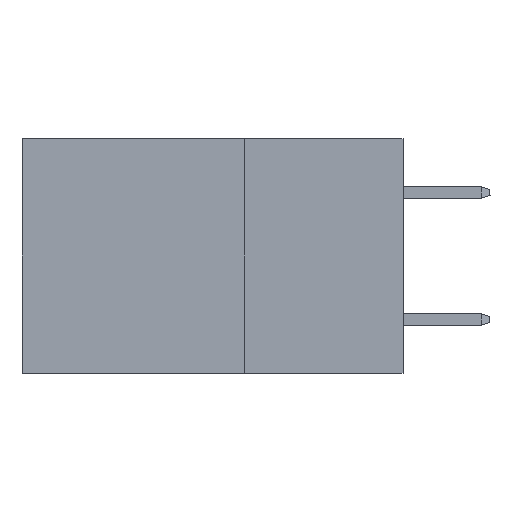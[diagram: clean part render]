
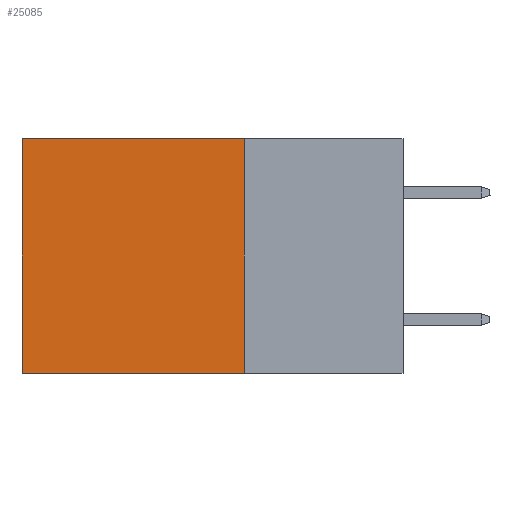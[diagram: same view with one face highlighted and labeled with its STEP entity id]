
A CAD part, left-side view. The second image highlights one B-rep face of the part: STEP entity #25085.
In plain terms, the highlighted planar face has unit normal (-1, 0, 0).
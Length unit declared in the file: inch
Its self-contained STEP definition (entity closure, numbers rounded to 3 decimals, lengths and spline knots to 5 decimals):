
#2461 = CARTESIAN_POINT ( 'NONE',  ( 0.2875, 0.6, -0.37 ) ) ;
#2779 = ORIENTED_EDGE ( 'NONE', *, *, #23482, .F. ) ;
#4397 = VERTEX_POINT ( 'NONE', #34480 ) ;
#4522 = DIRECTION ( 'NONE',  ( 0., 1., 0. ) ) ;
#4801 = CARTESIAN_POINT ( 'NONE',  ( 0.2875, 0.25, 0. ) ) ;
#5065 = LINE ( 'NONE', #26636, #22293 ) ;
#5544 = FACE_OUTER_BOUND ( 'NONE', #16501, .T. ) ;
#5665 = LINE ( 'NONE', #24556, #15319 ) ;
#6020 = CARTESIAN_POINT ( 'NONE',  ( 0.2875, 0.25, 0. ) ) ;
#7128 = VERTEX_POINT ( 'NONE', #9201 ) ;
#7500 = LINE ( 'NONE', #4801, #32509 ) ;
#9201 = CARTESIAN_POINT ( 'NONE',  ( 0.2875, 0.25, -0.37 ) ) ;
#9951 = ORIENTED_EDGE ( 'NONE', *, *, #18969, .F. ) ;
#11733 = ORIENTED_EDGE ( 'NONE', *, *, #13972, .T. ) ;
#11778 = VECTOR ( 'NONE', #14407, 39.37008 ) ;
#12647 = DIRECTION ( 'NONE',  ( 0., 0., -1. ) ) ;
#13736 = DIRECTION ( 'NONE',  ( 0., 0., -1. ) ) ;
#13972 = EDGE_CURVE ( 'NONE', #15903, #4397, #14052, .T. ) ;
#14052 = LINE ( 'NONE', #6020, #11778 ) ;
#14407 = DIRECTION ( 'NONE',  ( 0., 1., 0. ) ) ;
#15319 = VECTOR ( 'NONE', #16582, 39.37008 ) ;
#15903 = VERTEX_POINT ( 'NONE', #30292 ) ;
#16269 = PLANE ( 'NONE',  #17041 ) ;
#16460 = DIRECTION ( 'NONE',  ( 1., 0., 0. ) ) ;
#16501 = EDGE_LOOP ( 'NONE', ( #31914, #2779, #9951, #11733 ) ) ;
#16582 = DIRECTION ( 'NONE',  ( 0., 0., -1. ) ) ;
#17041 = AXIS2_PLACEMENT_3D ( 'NONE', #27297, #16460, #13736 ) ;
#18969 = EDGE_CURVE ( 'NONE', #15903, #7128, #7500, .T. ) ;
#22293 = VECTOR ( 'NONE', #4522, 39.37008 ) ;
#23482 = EDGE_CURVE ( 'NONE', #7128, #24217, #5065, .T. ) ;
#24217 = VERTEX_POINT ( 'NONE', #2461 ) ;
#24556 = CARTESIAN_POINT ( 'NONE',  ( 0.2875, 0.6, 0. ) ) ;
#25085 = ADVANCED_FACE ( 'NONE', ( #5544 ), #16269, .F. ) ;
#26636 = CARTESIAN_POINT ( 'NONE',  ( 0.2875, 0.25, -0.37 ) ) ;
#27297 = CARTESIAN_POINT ( 'NONE',  ( 0.2875, 0.25, 0. ) ) ;
#30292 = CARTESIAN_POINT ( 'NONE',  ( 0.2875, 0.25, 0. ) ) ;
#31505 = EDGE_CURVE ( 'NONE', #4397, #24217, #5665, .T. ) ;
#31914 = ORIENTED_EDGE ( 'NONE', *, *, #31505, .T. ) ;
#32509 = VECTOR ( 'NONE', #12647, 39.37008 ) ;
#34480 = CARTESIAN_POINT ( 'NONE',  ( 0.2875, 0.6, 0. ) ) ;
